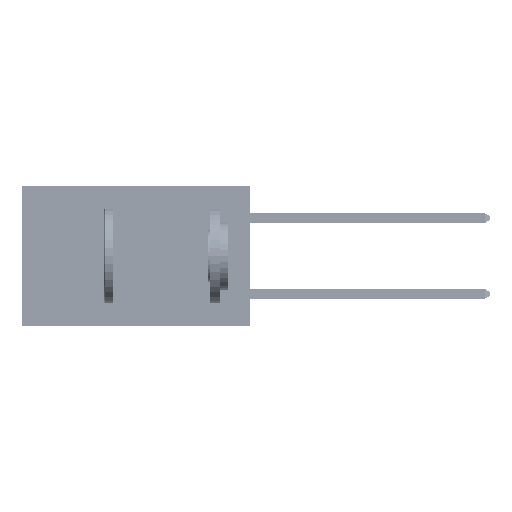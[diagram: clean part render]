
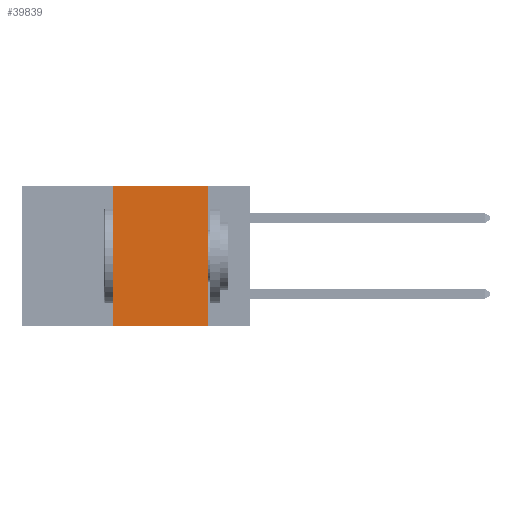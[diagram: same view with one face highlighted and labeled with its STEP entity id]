
A CAD part, left-side view. The second image highlights one B-rep face of the part: STEP entity #39839.
In plain terms, the highlighted planar face has unit normal (-1, 0, 0).
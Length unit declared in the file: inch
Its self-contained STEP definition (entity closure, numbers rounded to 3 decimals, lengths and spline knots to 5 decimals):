
#218 = CARTESIAN_POINT ( 'NONE',  ( 0., 0.6, -0.37 ) ) ;
#1639 = AXIS2_PLACEMENT_3D ( 'NONE', #6379, #31187, #25802 ) ;
#1652 = ORIENTED_EDGE ( 'NONE', *, *, #26082, .F. ) ;
#2416 = PLANE ( 'NONE',  #1639 ) ;
#2602 = VERTEX_POINT ( 'NONE', #16788 ) ;
#3075 = EDGE_CURVE ( 'NONE', #35680, #43783, #27874, .T. ) ;
#3556 = CARTESIAN_POINT ( 'NONE',  ( 0., 0.36, 0. ) ) ;
#4706 = DIRECTION ( 'NONE',  ( 0., -1., 0. ) ) ;
#6379 = CARTESIAN_POINT ( 'NONE',  ( 0., 0.6, 0. ) ) ;
#7166 = VECTOR ( 'NONE', #20467, 39.37008 ) ;
#11628 = CARTESIAN_POINT ( 'NONE',  ( 0., 0.36, 0. ) ) ;
#11640 = ORIENTED_EDGE ( 'NONE', *, *, #44603, .F. ) ;
#16788 = CARTESIAN_POINT ( 'NONE',  ( 0., 0.11, 0. ) ) ;
#16961 = VECTOR ( 'NONE', #4706, 39.37008 ) ;
#17433 = EDGE_CURVE ( 'NONE', #42339, #2602, #42246, .T. ) ;
#20467 = DIRECTION ( 'NONE',  ( 0., 0., 1. ) ) ;
#21370 = DIRECTION ( 'NONE',  ( 0., -1., 0. ) ) ;
#25802 = DIRECTION ( 'NONE',  ( 0., 0., -1. ) ) ;
#26082 = EDGE_CURVE ( 'NONE', #2602, #43783, #37247, .T. ) ;
#26996 = CARTESIAN_POINT ( 'NONE',  ( 0., 0.11, 0. ) ) ;
#27874 = LINE ( 'NONE', #218, #16961 ) ;
#28220 = VECTOR ( 'NONE', #43361, 39.37008 ) ;
#28554 = FACE_OUTER_BOUND ( 'NONE', #42073, .T. ) ;
#29381 = ORIENTED_EDGE ( 'NONE', *, *, #17433, .F. ) ;
#31187 = DIRECTION ( 'NONE',  ( 1., 0., 0. ) ) ;
#35680 = VERTEX_POINT ( 'NONE', #50819 ) ;
#37247 = LINE ( 'NONE', #26996, #28220 ) ;
#39839 = ADVANCED_FACE ( 'NONE', ( #28554 ), #2416, .F. ) ;
#42073 = EDGE_LOOP ( 'NONE', ( #1652, #29381, #11640, #42959 ) ) ;
#42246 = LINE ( 'NONE', #49953, #50005 ) ;
#42339 = VERTEX_POINT ( 'NONE', #11628 ) ;
#42959 = ORIENTED_EDGE ( 'NONE', *, *, #3075, .T. ) ;
#43361 = DIRECTION ( 'NONE',  ( 0., 0., -1. ) ) ;
#43783 = VERTEX_POINT ( 'NONE', #47982 ) ;
#44603 = EDGE_CURVE ( 'NONE', #35680, #42339, #51891, .T. ) ;
#47982 = CARTESIAN_POINT ( 'NONE',  ( 0., 0.11, -0.37 ) ) ;
#49953 = CARTESIAN_POINT ( 'NONE',  ( 0., 0.6, 0. ) ) ;
#50005 = VECTOR ( 'NONE', #21370, 39.37008 ) ;
#50819 = CARTESIAN_POINT ( 'NONE',  ( 0., 0.36, -0.37 ) ) ;
#51891 = LINE ( 'NONE', #3556, #7166 ) ;
